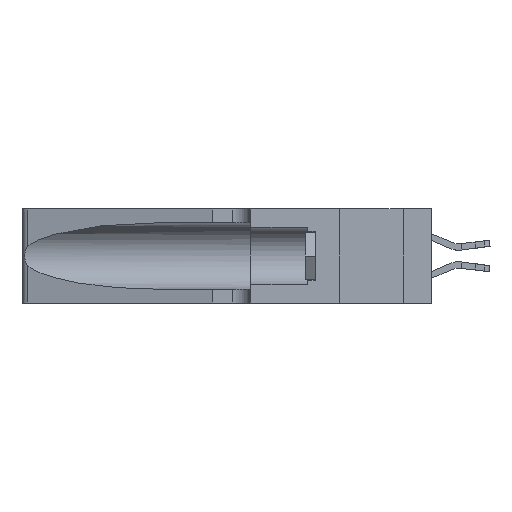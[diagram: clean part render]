
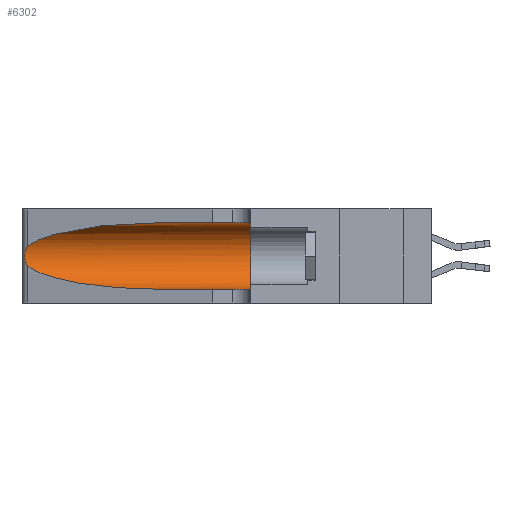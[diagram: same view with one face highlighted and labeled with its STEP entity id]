
A CAD part, left-side view. The second image highlights one B-rep face of the part: STEP entity #6302.
In plain terms, the highlighted cylindrical face has radius 3.308 mm (diameter 6.617 mm), a partial arc.
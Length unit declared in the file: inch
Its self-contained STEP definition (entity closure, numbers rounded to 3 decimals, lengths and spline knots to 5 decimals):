
#180 = VECTOR ( 'NONE', #6133, 39.37008 ) ;
#473 = CARTESIAN_POINT ( 'NONE',  ( 0.1305, 0.35, 0.31525 ) ) ;
#609 = FACE_OUTER_BOUND ( 'NONE', #20966, .T. ) ;
#1098 = EDGE_CURVE ( 'NONE', #4024, #12242, #22127, .T. ) ;
#1113 = CARTESIAN_POINT ( 'NONE',  ( 0.25487, 1.22718, 0.14631 ) ) ;
#1262 = CARTESIAN_POINT ( 'NONE',  ( 0.26075, 1.23896, 0.19203 ) ) ;
#1593 = EDGE_CURVE ( 'NONE', #19576, #20152, #11233, .T. ) ;
#1891 = DIRECTION ( 'NONE',  ( 0., 0., -1. ) ) ;
#3190 = CARTESIAN_POINT ( 'NONE',  ( 0.1305, 0.35, 0.185 ) ) ;
#3339 = CARTESIAN_POINT ( 'NONE',  ( 0.1305, 0.72297, 0.31525 ) ) ;
#4024 = VERTEX_POINT ( 'NONE', #3339 ) ;
#4829 = CARTESIAN_POINT ( 'NONE',  ( 0.25487, 1.22718, 0.22369 ) ) ;
#4959 = CARTESIAN_POINT ( 'NONE',  ( 0.1305, 0.72297, 0.05475 ) ) ;
#5141 = CARTESIAN_POINT ( 'NONE',  ( 0.2373, 1.15595, 0.08982 ) ) ;
#5258 = DIRECTION ( 'NONE',  ( 0., 0., 1. ) ) ;
#5299 = CARTESIAN_POINT ( 'NONE',  ( 0.25639, 1.23184, 0.21858 ) ) ;
#5384 = CARTESIAN_POINT ( 'NONE',  ( 0.25856, 1.23593, 0.16098 ) ) ;
#6133 = DIRECTION ( 'NONE',  ( 0., -1., 0. ) ) ;
#6275 = CARTESIAN_POINT ( 'NONE',  ( 0.25487, 1.22718, 0.22369 ) ) ;
#6302 = ADVANCED_FACE ( 'NONE', ( #609 ), #24561, .F. ) ;
#6367 = ORIENTED_EDGE ( 'NONE', *, *, #1098, .T. ) ;
#6721 = CARTESIAN_POINT ( 'NONE',  ( 0.2373, 1.15595, 0.28018 ) ) ;
#6722 = B_SPLINE_CURVE_WITH_KNOTS ( 'NONE', 3,
 ( #9475, #11603, #5299, #19581, #21658, #13503, #1262, #15563, #17627, #5384, #19667, #21755, #11517, #22348 ),
 .UNSPECIFIED., .F., .F.,
 ( 4, 2, 2, 2, 2, 2, 4 ),
 ( 0., 0.00027, 0.00053, 0.00107, 0.0016, 0.00187, 0.00214 ),
 .UNSPECIFIED. ) ;
#7106 = CARTESIAN_POINT ( 'NONE',  ( 0.18966, 0.96281, 0.05475 ) ) ;
#7684 = VERTEX_POINT ( 'NONE', #25371 ) ;
#8501 = LINE ( 'NONE', #22465, #180 ) ;
#9475 = CARTESIAN_POINT ( 'NONE',  ( 0.25487, 1.22718, 0.22369 ) ) ;
#9529 = AXIS2_PLACEMENT_3D ( 'NONE', #3190, #17594, #5258 ) ;
#9913 = CARTESIAN_POINT ( 'NONE',  ( 0.1305, 1.61858, 0.185 ) ) ;
#11233 = CIRCLE ( 'NONE', #9529, 0.13025 ) ;
#11334 = CARTESIAN_POINT ( 'NONE',  ( 0.25487, 1.22718, 0.14631 ) ) ;
#11517 = CARTESIAN_POINT ( 'NONE',  ( 0.25555, 1.22993, 0.14849 ) ) ;
#11603 = CARTESIAN_POINT ( 'NONE',  ( 0.25555, 1.22994, 0.2215 ) ) ;
#11816 = ORIENTED_EDGE ( 'NONE', *, *, #26139, .T. ) ;
#12024 = EDGE_CURVE ( 'NONE', #12242, #19907, #6722, .T. ) ;
#12068 = EDGE_CURVE ( 'NONE', #4024, #19576, #16860, .T. ) ;
#12242 = VERTEX_POINT ( 'NONE', #6275 ) ;
#12762 = CARTESIAN_POINT ( 'NONE',  ( 0.1305, 0.72297, 0.31525 ) ) ;
#13503 = CARTESIAN_POINT ( 'NONE',  ( 0.26018, 1.23835, 0.19895 ) ) ;
#14086 = ORIENTED_EDGE ( 'NONE', *, *, #1593, .F. ) ;
#14548 = ORIENTED_EDGE ( 'NONE', *, *, #12068, .F. ) ;
#15563 = CARTESIAN_POINT ( 'NONE',  ( 0.26075, 1.23896, 0.178 ) ) ;
#16181 = DIRECTION ( 'NONE',  ( 0., -1., 0. ) ) ;
#16860 = LINE ( 'NONE', #19937, #19429 ) ;
#16896 = CARTESIAN_POINT ( 'NONE',  ( 0.18966, 0.96281, 0.31525 ) ) ;
#17594 = DIRECTION ( 'NONE',  ( 0., 1., 0. ) ) ;
#17627 = CARTESIAN_POINT ( 'NONE',  ( 0.26017, 1.23833, 0.17102 ) ) ;
#18240 = CARTESIAN_POINT ( 'NONE',  ( 0.1305, 0.35, 0.05475 ) ) ;
#18822 =( BOUNDED_CURVE ( )  B_SPLINE_CURVE ( 3, ( #1113, #5141, #7106, #4959 ),
 .UNSPECIFIED., .F., .F. ) 
 B_SPLINE_CURVE_WITH_KNOTS ( ( 4, 4 ),
 ( 3.44316, 4.71239 ),
 .UNSPECIFIED. ) 
 CURVE ( )  GEOMETRIC_REPRESENTATION_ITEM ( )  RATIONAL_B_SPLINE_CURVE ( ( 1., 0.87, 0.87, 1. ) ) 
 REPRESENTATION_ITEM ( '' )  );
#19429 = VECTOR ( 'NONE', #16181, 39.37008 ) ;
#19576 = VERTEX_POINT ( 'NONE', #473 ) ;
#19581 = CARTESIAN_POINT ( 'NONE',  ( 0.25787, 1.23484, 0.2124 ) ) ;
#19611 = ORIENTED_EDGE ( 'NONE', *, *, #12024, .T. ) ;
#19667 = CARTESIAN_POINT ( 'NONE',  ( 0.25789, 1.23486, 0.15765 ) ) ;
#19907 = VERTEX_POINT ( 'NONE', #11334 ) ;
#19937 = CARTESIAN_POINT ( 'NONE',  ( 0.1305, 1.61858, 0.31525 ) ) ;
#20152 = VERTEX_POINT ( 'NONE', #18240 ) ;
#20966 = EDGE_LOOP ( 'NONE', ( #6367, #19611, #23909, #11816, #14086, #14548 ) ) ;
#21658 = CARTESIAN_POINT ( 'NONE',  ( 0.25854, 1.2359, 0.20912 ) ) ;
#21755 = CARTESIAN_POINT ( 'NONE',  ( 0.25639, 1.23186, 0.15144 ) ) ;
#22127 =( BOUNDED_CURVE ( )  B_SPLINE_CURVE ( 3, ( #12762, #16896, #6721, #4829 ),
 .UNSPECIFIED., .F., .F. ) 
 B_SPLINE_CURVE_WITH_KNOTS ( ( 4, 4 ),
 ( 1.5708, 2.84003 ),
 .UNSPECIFIED. ) 
 CURVE ( )  GEOMETRIC_REPRESENTATION_ITEM ( )  RATIONAL_B_SPLINE_CURVE ( ( 1., 0.87, 0.87, 1. ) ) 
 REPRESENTATION_ITEM ( '' )  );
#22348 = CARTESIAN_POINT ( 'NONE',  ( 0.25487, 1.22718, 0.14631 ) ) ;
#22465 = CARTESIAN_POINT ( 'NONE',  ( 0.1305, 1.61858, 0.05475 ) ) ;
#23179 = AXIS2_PLACEMENT_3D ( 'NONE', #9913, #24323, #1891 ) ;
#23909 = ORIENTED_EDGE ( 'NONE', *, *, #24108, .T. ) ;
#24108 = EDGE_CURVE ( 'NONE', #19907, #7684, #18822, .T. ) ;
#24323 = DIRECTION ( 'NONE',  ( 0., -1., 0. ) ) ;
#24561 = CYLINDRICAL_SURFACE ( 'NONE', #23179, 0.13025 ) ;
#25371 = CARTESIAN_POINT ( 'NONE',  ( 0.1305, 0.72297, 0.05475 ) ) ;
#26139 = EDGE_CURVE ( 'NONE', #7684, #20152, #8501, .T. ) ;
